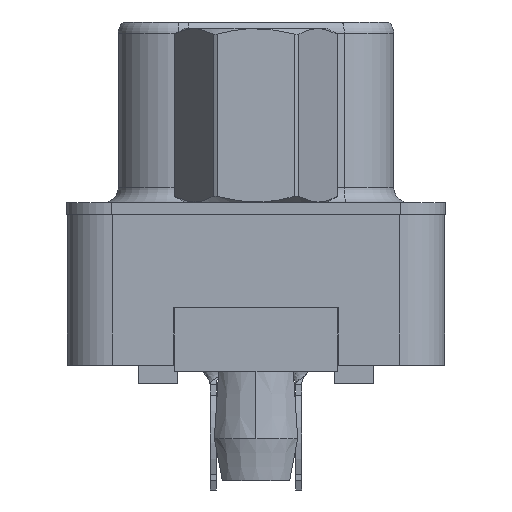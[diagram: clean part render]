
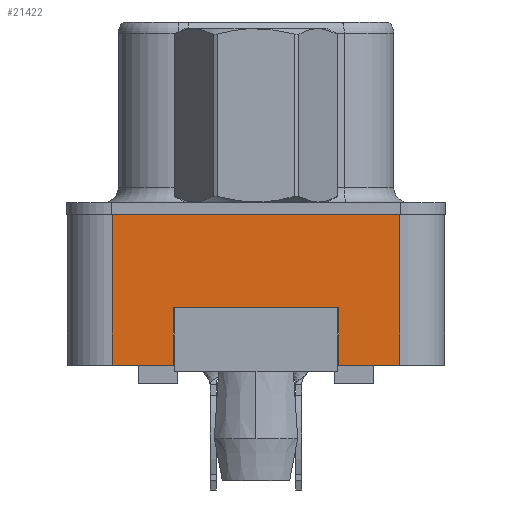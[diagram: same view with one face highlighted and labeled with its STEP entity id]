
A CAD part, left-side view. The second image highlights one B-rep face of the part: STEP entity #21422.
In plain terms, the highlighted planar face has unit normal (-1, 0, 0).
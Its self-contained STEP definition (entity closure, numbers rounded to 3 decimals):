
#509 = VERTEX_POINT ( 'NONE', #3891 ) ;
#561 = ORIENTED_EDGE ( 'NONE', *, *, #17712, .T. ) ;
#755 = EDGE_CURVE ( 'NONE', #27287, #11015, #34170, .T. ) ;
#757 = ORIENTED_EDGE ( 'NONE', *, *, #22735, .T. ) ;
#1570 = CARTESIAN_POINT ( 'NONE',  ( -2.91, -4.775, -5. ) ) ;
#2034 = CARTESIAN_POINT ( 'NONE',  ( -2.91, -2.75, -5. ) ) ;
#2217 = VERTEX_POINT ( 'NONE', #31351 ) ;
#2833 = VECTOR ( 'NONE', #22904, 1000. ) ;
#3276 = AXIS2_PLACEMENT_3D ( 'NONE', #12524, #23362, #34177 ) ;
#3413 = CARTESIAN_POINT ( 'NONE',  ( -2.91, 2.75, -3.1 ) ) ;
#3437 = CARTESIAN_POINT ( 'NONE',  ( -2.91, 2.75, -5. ) ) ;
#3891 = CARTESIAN_POINT ( 'NONE',  ( -2.91, -4.775, 0. ) ) ;
#4899 = VECTOR ( 'NONE', #20039, 1000. ) ;
#5096 = VERTEX_POINT ( 'NONE', #24051 ) ;
#5205 = EDGE_CURVE ( 'NONE', #7811, #2217, #30774, .T. ) ;
#7078 = ORIENTED_EDGE ( 'NONE', *, *, #21017, .T. ) ;
#7231 = DIRECTION ( 'NONE',  ( 0., -1., 0. ) ) ;
#7311 = CARTESIAN_POINT ( 'NONE',  ( -2.91, -4.775, -5. ) ) ;
#7400 = CARTESIAN_POINT ( 'NONE',  ( -2.91, -4.775, 0. ) ) ;
#7791 = VERTEX_POINT ( 'NONE', #7311 ) ;
#7811 = VERTEX_POINT ( 'NONE', #27516 ) ;
#11015 = VERTEX_POINT ( 'NONE', #3437 ) ;
#12210 = LINE ( 'NONE', #23049, #35014 ) ;
#12285 = LINE ( 'NONE', #34131, #18936 ) ;
#12384 = LINE ( 'NONE', #7400, #29694 ) ;
#12524 = CARTESIAN_POINT ( 'NONE',  ( -2.91, -4.775, -5. ) ) ;
#12926 = VERTEX_POINT ( 'NONE', #2034 ) ;
#13556 = ORIENTED_EDGE ( 'NONE', *, *, #13841, .F. ) ;
#13841 = EDGE_CURVE ( 'NONE', #2217, #509, #12384, .T. ) ;
#14760 = EDGE_CURVE ( 'NONE', #5096, #27287, #12285, .T. ) ;
#14906 = LINE ( 'NONE', #1570, #2833 ) ;
#16051 = VECTOR ( 'NONE', #31345, 1000. ) ;
#16806 = DIRECTION ( 'NONE',  ( 0., 0., 1. ) ) ;
#17366 = CARTESIAN_POINT ( 'NONE',  ( -2.91, -2.75, -3.1 ) ) ;
#17494 = PLANE ( 'NONE',  #3276 ) ;
#17712 = EDGE_CURVE ( 'NONE', #5096, #12926, #22709, .T. ) ;
#18231 = DIRECTION ( 'NONE',  ( 0., -1., 0. ) ) ;
#18936 = VECTOR ( 'NONE', #23134, 1000. ) ;
#20000 = EDGE_LOOP ( 'NONE', ( #561, #27332, #757, #13556, #26649, #7078, #20413, #29571 ) ) ;
#20039 = DIRECTION ( 'NONE',  ( 0., 0., -1. ) ) ;
#20062 = VECTOR ( 'NONE', #30612, 1000. ) ;
#20413 = ORIENTED_EDGE ( 'NONE', *, *, #755, .F. ) ;
#21017 = EDGE_CURVE ( 'NONE', #7811, #11015, #12210, .T. ) ;
#21422 = ADVANCED_FACE ( 'NONE', ( #28511 ), #17494, .T. ) ;
#22435 = CARTESIAN_POINT ( 'NONE',  ( -2.91, 4.775, -5. ) ) ;
#22709 = LINE ( 'NONE', #17366, #4899 ) ;
#22735 = EDGE_CURVE ( 'NONE', #7791, #509, #32975, .T. ) ;
#22904 = DIRECTION ( 'NONE',  ( 0., -1., 0. ) ) ;
#23049 = CARTESIAN_POINT ( 'NONE',  ( -2.91, -4.775, -5. ) ) ;
#23134 = DIRECTION ( 'NONE',  ( 0., 1., 0. ) ) ;
#23362 = DIRECTION ( 'NONE',  ( -1., 0., 0. ) ) ;
#24051 = CARTESIAN_POINT ( 'NONE',  ( -2.91, -2.75, -3.1 ) ) ;
#26649 = ORIENTED_EDGE ( 'NONE', *, *, #5205, .F. ) ;
#27188 = VECTOR ( 'NONE', #16806, 1000. ) ;
#27287 = VERTEX_POINT ( 'NONE', #3413 ) ;
#27332 = ORIENTED_EDGE ( 'NONE', *, *, #31035, .T. ) ;
#27516 = CARTESIAN_POINT ( 'NONE',  ( -2.91, 4.775, -5. ) ) ;
#28147 = CARTESIAN_POINT ( 'NONE',  ( -2.91, 2.75, -3.1 ) ) ;
#28511 = FACE_OUTER_BOUND ( 'NONE', #20000, .T. ) ;
#29571 = ORIENTED_EDGE ( 'NONE', *, *, #14760, .F. ) ;
#29694 = VECTOR ( 'NONE', #18231, 1000. ) ;
#30612 = DIRECTION ( 'NONE',  ( 0., 0., 1. ) ) ;
#30774 = LINE ( 'NONE', #22435, #20062 ) ;
#31035 = EDGE_CURVE ( 'NONE', #12926, #7791, #14906, .T. ) ;
#31345 = DIRECTION ( 'NONE',  ( 0., 0., -1. ) ) ;
#31351 = CARTESIAN_POINT ( 'NONE',  ( -2.91, 4.775, 0. ) ) ;
#32975 = LINE ( 'NONE', #33143, #27188 ) ;
#33143 = CARTESIAN_POINT ( 'NONE',  ( -2.91, -4.775, -5. ) ) ;
#34131 = CARTESIAN_POINT ( 'NONE',  ( -2.91, 2.75, -3.1 ) ) ;
#34170 = LINE ( 'NONE', #28147, #16051 ) ;
#34177 = DIRECTION ( 'NONE',  ( 0., 0., 1. ) ) ;
#35014 = VECTOR ( 'NONE', #7231, 1000. ) ;
